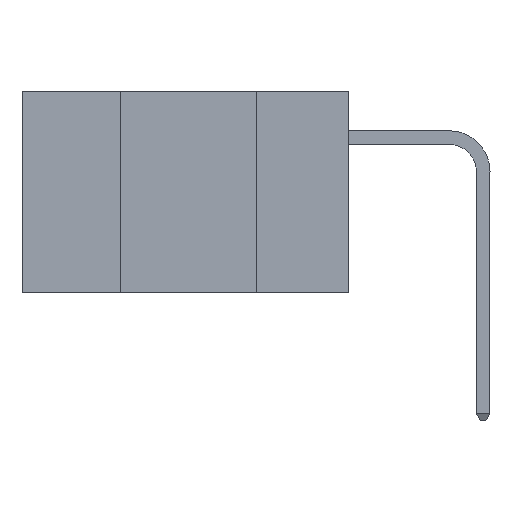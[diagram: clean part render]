
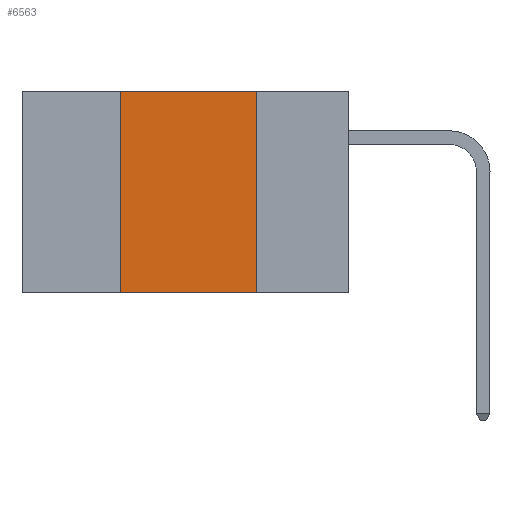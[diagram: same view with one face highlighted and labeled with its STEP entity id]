
A CAD part, left-side view. The second image highlights one B-rep face of the part: STEP entity #6563.
In plain terms, the highlighted planar face has unit normal (-1, 0, 0).
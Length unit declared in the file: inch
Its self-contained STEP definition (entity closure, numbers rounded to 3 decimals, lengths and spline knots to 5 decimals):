
#492 = VECTOR ( 'NONE', #4393, 39.37008 ) ;
#1061 = DIRECTION ( 'NONE',  ( 0., -1., 0. ) ) ;
#1268 = PLANE ( 'NONE',  #11041 ) ;
#1350 = CARTESIAN_POINT ( 'NONE',  ( 0., 0.6, 0. ) ) ;
#1621 = VERTEX_POINT ( 'NONE', #13009 ) ;
#2646 = EDGE_CURVE ( 'NONE', #1621, #13218, #4941, .T. ) ;
#2826 = VECTOR ( 'NONE', #14167, 39.37008 ) ;
#4393 = DIRECTION ( 'NONE',  ( 0., 0., 1. ) ) ;
#4941 = LINE ( 'NONE', #5361, #13706 ) ;
#4953 = DIRECTION ( 'NONE',  ( 0., 0., -1. ) ) ;
#5361 = CARTESIAN_POINT ( 'NONE',  ( 0., 0.6, -0.37 ) ) ;
#6563 = ADVANCED_FACE ( 'NONE', ( #15444 ), #1268, .F. ) ;
#7177 = DIRECTION ( 'NONE',  ( 0., -1., 0. ) ) ;
#8136 = CARTESIAN_POINT ( 'NONE',  ( 0., 0.6, 0. ) ) ;
#8863 = CARTESIAN_POINT ( 'NONE',  ( 0., 0.17, 0. ) ) ;
#9386 = LINE ( 'NONE', #14849, #492 ) ;
#10748 = ORIENTED_EDGE ( 'NONE', *, *, #13762, .F. ) ;
#10876 = VERTEX_POINT ( 'NONE', #8863 ) ;
#11041 = AXIS2_PLACEMENT_3D ( 'NONE', #1350, #15390, #4953 ) ;
#11305 = ORIENTED_EDGE ( 'NONE', *, *, #12747, .F. ) ;
#11689 = LINE ( 'NONE', #14240, #2826 ) ;
#12391 = ORIENTED_EDGE ( 'NONE', *, *, #15544, .F. ) ;
#12747 = EDGE_CURVE ( 'NONE', #21248, #10876, #19992, .T. ) ;
#13009 = CARTESIAN_POINT ( 'NONE',  ( 0., 0.42, -0.37 ) ) ;
#13218 = VERTEX_POINT ( 'NONE', #14496 ) ;
#13706 = VECTOR ( 'NONE', #7177, 39.37008 ) ;
#13762 = EDGE_CURVE ( 'NONE', #10876, #13218, #11689, .T. ) ;
#14167 = DIRECTION ( 'NONE',  ( 0., 0., -1. ) ) ;
#14240 = CARTESIAN_POINT ( 'NONE',  ( 0., 0.17, 0. ) ) ;
#14496 = CARTESIAN_POINT ( 'NONE',  ( 0., 0.17, -0.37 ) ) ;
#14849 = CARTESIAN_POINT ( 'NONE',  ( 0., 0.42, 0. ) ) ;
#14936 = VECTOR ( 'NONE', #1061, 39.37008 ) ;
#15390 = DIRECTION ( 'NONE',  ( 1., 0., 0. ) ) ;
#15444 = FACE_OUTER_BOUND ( 'NONE', #19554, .T. ) ;
#15544 = EDGE_CURVE ( 'NONE', #1621, #21248, #9386, .T. ) ;
#17500 = CARTESIAN_POINT ( 'NONE',  ( 0., 0.42, 0. ) ) ;
#19554 = EDGE_LOOP ( 'NONE', ( #10748, #11305, #12391, #21961 ) ) ;
#19992 = LINE ( 'NONE', #8136, #14936 ) ;
#21248 = VERTEX_POINT ( 'NONE', #17500 ) ;
#21961 = ORIENTED_EDGE ( 'NONE', *, *, #2646, .T. ) ;
